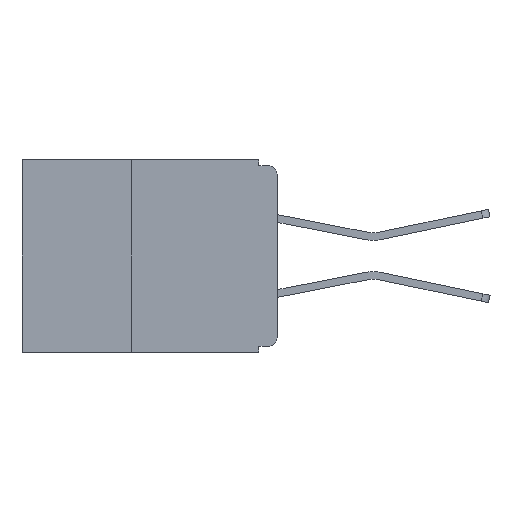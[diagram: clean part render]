
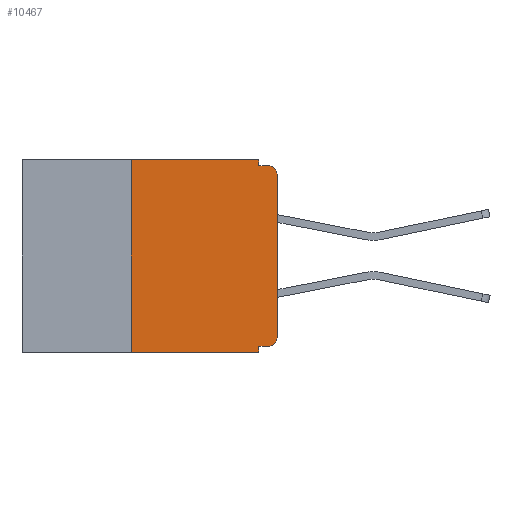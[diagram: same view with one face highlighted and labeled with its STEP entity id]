
A CAD part, left-side view. The second image highlights one B-rep face of the part: STEP entity #10467.
In plain terms, the highlighted planar face has unit normal (-1, 0, 0).
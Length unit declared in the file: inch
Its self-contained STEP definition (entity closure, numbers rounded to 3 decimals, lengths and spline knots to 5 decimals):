
#154 = LINE ( 'NONE', #15929, #16933 ) ;
#245 = VERTEX_POINT ( 'NONE', #11803 ) ;
#297 = VERTEX_POINT ( 'NONE', #20547 ) ;
#949 = LINE ( 'NONE', #15550, #17187 ) ;
#1175 = VERTEX_POINT ( 'NONE', #9486 ) ;
#1606 = LINE ( 'NONE', #12853, #18781 ) ;
#2051 = ORIENTED_EDGE ( 'NONE', *, *, #11662, .F. ) ;
#2332 = ORIENTED_EDGE ( 'NONE', *, *, #7085, .F. ) ;
#2721 = EDGE_CURVE ( 'NONE', #11254, #245, #4441, .T. ) ;
#2782 = AXIS2_PLACEMENT_3D ( 'NONE', #7989, #8544, #8562 ) ;
#2852 = CARTESIAN_POINT ( 'NONE',  ( 0., 0.031, -0.33 ) ) ;
#3076 = DIRECTION ( 'NONE',  ( 0., -1., 0. ) ) ;
#3180 = DIRECTION ( 'NONE',  ( 0., -1., 0. ) ) ;
#3182 = ORIENTED_EDGE ( 'NONE', *, *, #12244, .F. ) ;
#3285 = AXIS2_PLACEMENT_3D ( 'NONE', #18912, #9402, #20509 ) ;
#3476 = VERTEX_POINT ( 'NONE', #17606 ) ;
#3599 = DIRECTION ( 'NONE',  ( 0., 0., 1. ) ) ;
#3602 = ORIENTED_EDGE ( 'NONE', *, *, #11594, .F. ) ;
#4441 = CIRCLE ( 'NONE', #2782, 0.015 ) ;
#4897 = LINE ( 'NONE', #11242, #15259 ) ;
#5170 = EDGE_CURVE ( 'NONE', #297, #8791, #949, .T. ) ;
#5550 = LINE ( 'NONE', #9830, #13606 ) ;
#6237 = DIRECTION ( 'NONE',  ( 0., -1., 0. ) ) ;
#6933 = CARTESIAN_POINT ( 'NONE',  ( 0., 0., -0.025 ) ) ;
#7085 = EDGE_CURVE ( 'NONE', #17480, #297, #5550, .T. ) ;
#7359 = ORIENTED_EDGE ( 'NONE', *, *, #5170, .F. ) ;
#7818 = ORIENTED_EDGE ( 'NONE', *, *, #20342, .T. ) ;
#7868 = VERTEX_POINT ( 'NONE', #19728 ) ;
#7989 = CARTESIAN_POINT ( 'NONE',  ( 0., 0.015, -0.025 ) ) ;
#8348 = VECTOR ( 'NONE', #3599, 39.37008 ) ;
#8465 = EDGE_CURVE ( 'NONE', #3476, #20854, #12577, .T. ) ;
#8497 = ORIENTED_EDGE ( 'NONE', *, *, #8465, .F. ) ;
#8544 = DIRECTION ( 'NONE',  ( -1., 0., 0. ) ) ;
#8562 = DIRECTION ( 'NONE',  ( 0., 0., -1. ) ) ;
#8791 = VERTEX_POINT ( 'NONE', #2852 ) ;
#9402 = DIRECTION ( 'NONE',  ( -1., 0., 0. ) ) ;
#9486 = CARTESIAN_POINT ( 'NONE',  ( 0., 0.031, -0.01 ) ) ;
#9544 = EDGE_CURVE ( 'NONE', #3476, #8791, #1606, .T. ) ;
#9567 = VERTEX_POINT ( 'NONE', #19041 ) ;
#9773 = CARTESIAN_POINT ( 'NONE',  ( 0., 0.437, 0. ) ) ;
#9830 = CARTESIAN_POINT ( 'NONE',  ( 0., 0., -0.32 ) ) ;
#10128 = EDGE_CURVE ( 'NONE', #9567, #11254, #15825, .T. ) ;
#10467 = ADVANCED_FACE ( 'NONE', ( #13529 ), #17703, .F. ) ;
#10565 = DIRECTION ( 'NONE',  ( 0., 0., 1. ) ) ;
#10655 = CARTESIAN_POINT ( 'NONE',  ( 0., 0.25, 0. ) ) ;
#10800 = ORIENTED_EDGE ( 'NONE', *, *, #2721, .T. ) ;
#11242 = CARTESIAN_POINT ( 'NONE',  ( 0., 0.031, 0. ) ) ;
#11254 = VERTEX_POINT ( 'NONE', #6933 ) ;
#11367 = DIRECTION ( 'NONE',  ( 0., 0., -1. ) ) ;
#11418 = DIRECTION ( 'NONE',  ( 0., 1., 0. ) ) ;
#11594 = EDGE_CURVE ( 'NONE', #20854, #7868, #17214, .T. ) ;
#11662 = EDGE_CURVE ( 'NONE', #7868, #1175, #4897, .T. ) ;
#11803 = CARTESIAN_POINT ( 'NONE',  ( 0., 0.015, -0.01 ) ) ;
#12244 = EDGE_CURVE ( 'NONE', #1175, #245, #154, .T. ) ;
#12361 = CARTESIAN_POINT ( 'NONE',  ( 0., 0.015, -0.32 ) ) ;
#12577 = LINE ( 'NONE', #13330, #8348 ) ;
#12737 = AXIS2_PLACEMENT_3D ( 'NONE', #9773, #20864, #11367 ) ;
#12853 = CARTESIAN_POINT ( 'NONE',  ( 0., 0.437, -0.33 ) ) ;
#13330 = CARTESIAN_POINT ( 'NONE',  ( 0., 0.25, -0.33 ) ) ;
#13529 = FACE_OUTER_BOUND ( 'NONE', #15289, .T. ) ;
#13606 = VECTOR ( 'NONE', #11418, 39.37008 ) ;
#13780 = ORIENTED_EDGE ( 'NONE', *, *, #9544, .T. ) ;
#14264 = CARTESIAN_POINT ( 'NONE',  ( 0., 0.437, 0. ) ) ;
#15259 = VECTOR ( 'NONE', #17658, 39.37008 ) ;
#15289 = EDGE_LOOP ( 'NONE', ( #15803, #10800, #3182, #2051, #3602, #8497, #13780, #7359, #2332, #7818 ) ) ;
#15328 = CARTESIAN_POINT ( 'NONE',  ( 0., 0., 0. ) ) ;
#15550 = CARTESIAN_POINT ( 'NONE',  ( 0., 0.031, -0.33 ) ) ;
#15803 = ORIENTED_EDGE ( 'NONE', *, *, #10128, .T. ) ;
#15825 = LINE ( 'NONE', #15328, #19492 ) ;
#15929 = CARTESIAN_POINT ( 'NONE',  ( 0., 0., -0.01 ) ) ;
#16933 = VECTOR ( 'NONE', #3076, 39.37008 ) ;
#17121 = DIRECTION ( 'NONE',  ( 0., 0., -1. ) ) ;
#17187 = VECTOR ( 'NONE', #17121, 39.37008 ) ;
#17214 = LINE ( 'NONE', #14264, #17704 ) ;
#17480 = VERTEX_POINT ( 'NONE', #12361 ) ;
#17606 = CARTESIAN_POINT ( 'NONE',  ( 0., 0.25, -0.33 ) ) ;
#17658 = DIRECTION ( 'NONE',  ( 0., 0., -1. ) ) ;
#17703 = PLANE ( 'NONE',  #12737 ) ;
#17704 = VECTOR ( 'NONE', #6237, 39.37008 ) ;
#18059 = CIRCLE ( 'NONE', #3285, 0.015 ) ;
#18781 = VECTOR ( 'NONE', #3180, 39.37008 ) ;
#18912 = CARTESIAN_POINT ( 'NONE',  ( 0., 0.015, -0.305 ) ) ;
#19041 = CARTESIAN_POINT ( 'NONE',  ( 0., 0., -0.305 ) ) ;
#19492 = VECTOR ( 'NONE', #10565, 39.37008 ) ;
#19728 = CARTESIAN_POINT ( 'NONE',  ( 0., 0.031, 0. ) ) ;
#20342 = EDGE_CURVE ( 'NONE', #17480, #9567, #18059, .T. ) ;
#20509 = DIRECTION ( 'NONE',  ( 0., 0., -1. ) ) ;
#20547 = CARTESIAN_POINT ( 'NONE',  ( 0., 0.031, -0.32 ) ) ;
#20854 = VERTEX_POINT ( 'NONE', #10655 ) ;
#20864 = DIRECTION ( 'NONE',  ( 1., 0., 0. ) ) ;
